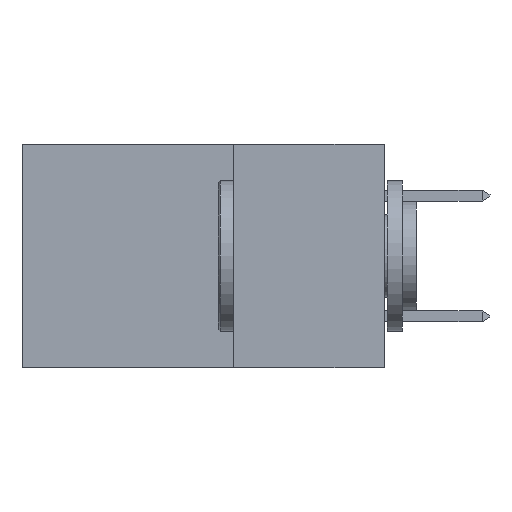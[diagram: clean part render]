
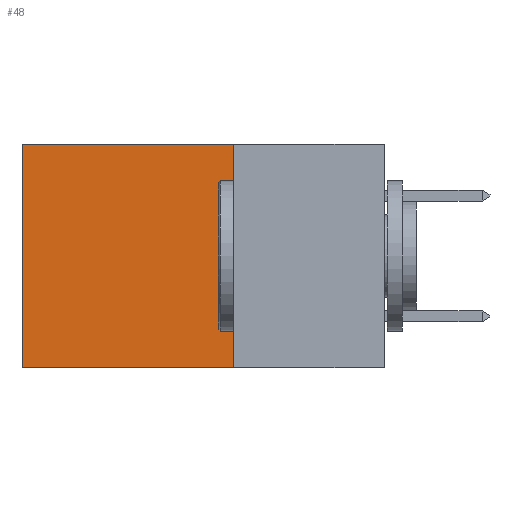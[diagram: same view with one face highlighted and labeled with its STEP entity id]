
A CAD part, left-side view. The second image highlights one B-rep face of the part: STEP entity #48.
In plain terms, the highlighted planar face has unit normal (-1, 0, 0).
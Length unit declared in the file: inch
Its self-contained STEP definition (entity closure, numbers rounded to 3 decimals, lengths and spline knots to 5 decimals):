
#48 = ADVANCED_FACE ( 'NONE', ( #784 ), #16886, .F. ) ;
#585 = CARTESIAN_POINT ( 'NONE',  ( 0.2875, 0.25, -0.37 ) ) ;
#597 = ORIENTED_EDGE ( 'NONE', *, *, #24617, .T. ) ;
#784 = FACE_OUTER_BOUND ( 'NONE', #7402, .T. ) ;
#838 = DIRECTION ( 'NONE',  ( 0., 0., -1. ) ) ;
#2391 = VERTEX_POINT ( 'NONE', #20908 ) ;
#4127 = LINE ( 'NONE', #23509, #8043 ) ;
#4295 = EDGE_CURVE ( 'NONE', #22415, #5058, #4127, .T. ) ;
#4551 = CARTESIAN_POINT ( 'NONE',  ( 0.2875, 0.6, 0. ) ) ;
#4636 = VERTEX_POINT ( 'NONE', #9758 ) ;
#5058 = VERTEX_POINT ( 'NONE', #11251 ) ;
#5377 = ORIENTED_EDGE ( 'NONE', *, *, #20647, .T. ) ;
#7114 = ORIENTED_EDGE ( 'NONE', *, *, #10156, .F. ) ;
#7402 = EDGE_LOOP ( 'NONE', ( #5377, #19312, #7114, #597 ) ) ;
#8043 = VECTOR ( 'NONE', #14483, 39.37008 ) ;
#9758 = CARTESIAN_POINT ( 'NONE',  ( 0.2875, 0.25, 0. ) ) ;
#10156 = EDGE_CURVE ( 'NONE', #4636, #22415, #14657, .T. ) ;
#10924 = CARTESIAN_POINT ( 'NONE',  ( 0.2875, 0.25, 0. ) ) ;
#11251 = CARTESIAN_POINT ( 'NONE',  ( 0.2875, 0.6, -0.37 ) ) ;
#13569 = VECTOR ( 'NONE', #23102, 39.37008 ) ;
#13575 = LINE ( 'NONE', #4551, #13866 ) ;
#13724 = AXIS2_PLACEMENT_3D ( 'NONE', #22740, #18569, #24250 ) ;
#13866 = VECTOR ( 'NONE', #838, 39.37008 ) ;
#14483 = DIRECTION ( 'NONE',  ( 0., 1., 0. ) ) ;
#14657 = LINE ( 'NONE', #10924, #19440 ) ;
#16886 = PLANE ( 'NONE',  #13724 ) ;
#18569 = DIRECTION ( 'NONE',  ( 1., 0., 0. ) ) ;
#19015 = CARTESIAN_POINT ( 'NONE',  ( 0.2875, 0.25, 0. ) ) ;
#19312 = ORIENTED_EDGE ( 'NONE', *, *, #4295, .F. ) ;
#19440 = VECTOR ( 'NONE', #22209, 39.37008 ) ;
#20647 = EDGE_CURVE ( 'NONE', #2391, #5058, #13575, .T. ) ;
#20908 = CARTESIAN_POINT ( 'NONE',  ( 0.2875, 0.6, 0. ) ) ;
#22209 = DIRECTION ( 'NONE',  ( 0., 0., -1. ) ) ;
#22415 = VERTEX_POINT ( 'NONE', #585 ) ;
#22740 = CARTESIAN_POINT ( 'NONE',  ( 0.2875, 0.25, 0. ) ) ;
#22826 = LINE ( 'NONE', #19015, #13569 ) ;
#23102 = DIRECTION ( 'NONE',  ( 0., 1., 0. ) ) ;
#23509 = CARTESIAN_POINT ( 'NONE',  ( 0.2875, 0.25, -0.37 ) ) ;
#24250 = DIRECTION ( 'NONE',  ( 0., 0., -1. ) ) ;
#24617 = EDGE_CURVE ( 'NONE', #4636, #2391, #22826, .T. ) ;
